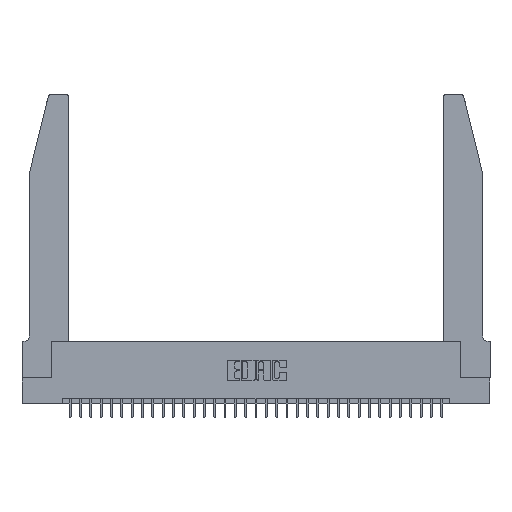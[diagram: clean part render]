
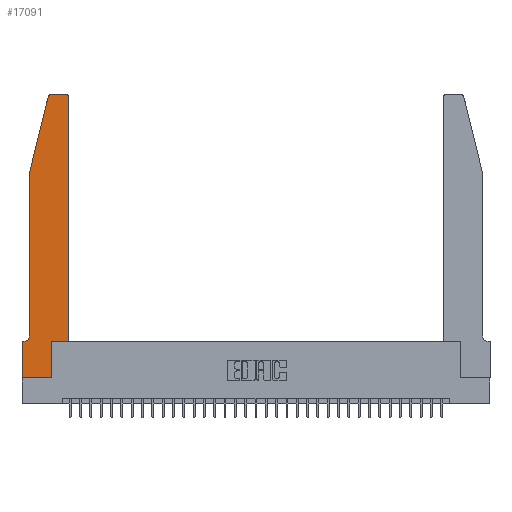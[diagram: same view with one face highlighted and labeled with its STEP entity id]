
A CAD part, top view. The second image highlights one B-rep face of the part: STEP entity #17091.
In plain terms, the highlighted planar face has unit normal (0, 0, 1).
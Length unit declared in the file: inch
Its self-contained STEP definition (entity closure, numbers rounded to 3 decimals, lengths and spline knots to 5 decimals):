
#749 = LINE ( 'NONE', #29789, #25771 ) ;
#884 = PLANE ( 'NONE',  #28031 ) ;
#921 = CARTESIAN_POINT ( 'NONE',  ( 0.4205, 2.72, 0.37 ) ) ;
#1233 = DIRECTION ( 'NONE',  ( 0., 0., 1. ) ) ;
#1353 = VECTOR ( 'NONE', #1467, 39.37008 ) ;
#1467 = DIRECTION ( 'NONE',  ( 0., -1., 0. ) ) ;
#1712 = ORIENTED_EDGE ( 'NONE', *, *, #6478, .T. ) ;
#1741 = CARTESIAN_POINT ( 'NONE',  ( 0., 0., 0.37 ) ) ;
#2584 = VERTEX_POINT ( 'NONE', #10958 ) ;
#2595 = ORIENTED_EDGE ( 'NONE', *, *, #30237, .T. ) ;
#3160 = VECTOR ( 'NONE', #19468, 39.37008 ) ;
#4023 = VERTEX_POINT ( 'NONE', #29581 ) ;
#4165 = ORIENTED_EDGE ( 'NONE', *, *, #14475, .T. ) ;
#5285 = VECTOR ( 'NONE', #31434, 39.37008 ) ;
#5296 = CARTESIAN_POINT ( 'NONE',  ( 0.4505, 0.35, 0.37 ) ) ;
#5356 = LINE ( 'NONE', #7424, #5285 ) ;
#5617 = ORIENTED_EDGE ( 'NONE', *, *, #32740, .T. ) ;
#5955 = VERTEX_POINT ( 'NONE', #13078 ) ;
#6478 = EDGE_CURVE ( 'NONE', #10735, #11610, #31607, .T. ) ;
#6593 = CIRCLE ( 'NONE', #11052, 0.07 ) ;
#6768 = CARTESIAN_POINT ( 'NONE',  ( 0.0755, 2., 0.37 ) ) ;
#6845 = ORIENTED_EDGE ( 'NONE', *, *, #18375, .T. ) ;
#7424 = CARTESIAN_POINT ( 'NONE',  ( 0., 0., 0.37 ) ) ;
#8068 = EDGE_CURVE ( 'NONE', #25461, #2584, #25272, .T. ) ;
#8406 = CARTESIAN_POINT ( 'NONE',  ( 0., 0., 0.37 ) ) ;
#8772 = LINE ( 'NONE', #8406, #3160 ) ;
#8917 = DIRECTION ( 'NONE',  ( 0., 0., 1. ) ) ;
#9054 = CARTESIAN_POINT ( 'NONE',  ( 0.2865, 0.35, 0.37 ) ) ;
#9136 = ORIENTED_EDGE ( 'NONE', *, *, #8068, .T. ) ;
#9634 = DIRECTION ( 'NONE',  ( 0., 0., -1. ) ) ;
#10425 = LINE ( 'NONE', #21261, #24882 ) ;
#10735 = VERTEX_POINT ( 'NONE', #19805 ) ;
#10795 = EDGE_CURVE ( 'NONE', #16302, #22369, #6593, .T. ) ;
#10958 = CARTESIAN_POINT ( 'NONE',  ( 0.25487, 2.72718, 0.37 ) ) ;
#11052 = AXIS2_PLACEMENT_3D ( 'NONE', #12244, #9634, #22392 ) ;
#11101 = VERTEX_POINT ( 'NONE', #6768 ) ;
#11190 = CARTESIAN_POINT ( 'NONE',  ( 0.4205, 2.75, 0.37 ) ) ;
#11448 = VECTOR ( 'NONE', #24638, 39.37008 ) ;
#11577 = DIRECTION ( 'NONE',  ( 0., 0., 1. ) ) ;
#11610 = VERTEX_POINT ( 'NONE', #11190 ) ;
#12244 = CARTESIAN_POINT ( 'NONE',  ( 0.0055, 0.42, 0.37 ) ) ;
#12999 = LINE ( 'NONE', #5296, #15747 ) ;
#13078 = CARTESIAN_POINT ( 'NONE',  ( 0.2865, 0., 0.37 ) ) ;
#14475 = EDGE_CURVE ( 'NONE', #26114, #4023, #12999, .T. ) ;
#14532 = DIRECTION ( 'NONE',  ( 1., 0., 0. ) ) ;
#15346 = EDGE_CURVE ( 'NONE', #22369, #16473, #23579, .T. ) ;
#15747 = VECTOR ( 'NONE', #31720, 39.37008 ) ;
#16057 = CARTESIAN_POINT ( 'NONE',  ( 0.0755, 0.42, 0.37 ) ) ;
#16302 = VERTEX_POINT ( 'NONE', #16057 ) ;
#16473 = VERTEX_POINT ( 'NONE', #32996 ) ;
#16662 = EDGE_CURVE ( 'NONE', #5955, #26114, #749, .T. ) ;
#17091 = ADVANCED_FACE ( 'NONE', ( #32904 ), #884, .T. ) ;
#17492 = DIRECTION ( 'NONE',  ( 1., 0., 0. ) ) ;
#17626 = ORIENTED_EDGE ( 'NONE', *, *, #29405, .T. ) ;
#18089 = AXIS2_PLACEMENT_3D ( 'NONE', #921, #11577, #30134 ) ;
#18313 = ORIENTED_EDGE ( 'NONE', *, *, #16662, .T. ) ;
#18375 = EDGE_CURVE ( 'NONE', #2584, #11101, #32875, .T. ) ;
#18906 = CARTESIAN_POINT ( 'NONE',  ( 0.4505, 0.35, 0.37 ) ) ;
#19468 = DIRECTION ( 'NONE',  ( 1., 0., 0. ) ) ;
#19798 = EDGE_CURVE ( 'NONE', #11101, #16302, #28036, .T. ) ;
#19805 = CARTESIAN_POINT ( 'NONE',  ( 0.4505, 2.72, 0.37 ) ) ;
#20952 = DIRECTION ( 'NONE',  ( -1., 0., 0. ) ) ;
#21128 = CARTESIAN_POINT ( 'NONE',  ( 0.0755, 0.35, 0.37 ) ) ;
#21261 = CARTESIAN_POINT ( 'NONE',  ( 0.2605, 2.75, 0.37 ) ) ;
#22349 = DIRECTION ( 'NONE',  ( -0.239, -0.971, 0. ) ) ;
#22369 = VERTEX_POINT ( 'NONE', #28706 ) ;
#22392 = DIRECTION ( 'NONE',  ( -1., 0., 0. ) ) ;
#23579 = LINE ( 'NONE', #21128, #25237 ) ;
#24131 = LINE ( 'NONE', #18906, #11448 ) ;
#24638 = DIRECTION ( 'NONE',  ( 0., 1., 0. ) ) ;
#24882 = VECTOR ( 'NONE', #34420, 39.37008 ) ;
#25176 = CARTESIAN_POINT ( 'NONE',  ( 0.284, 2.72, 0.37 ) ) ;
#25237 = VECTOR ( 'NONE', #20952, 39.37008 ) ;
#25239 = CARTESIAN_POINT ( 'NONE',  ( 0.0755, 2., 0.37 ) ) ;
#25272 = CIRCLE ( 'NONE', #29747, 0.03 ) ;
#25461 = VERTEX_POINT ( 'NONE', #30428 ) ;
#25683 = ORIENTED_EDGE ( 'NONE', *, *, #15346, .T. ) ;
#25771 = VECTOR ( 'NONE', #26799, 39.37008 ) ;
#26114 = VERTEX_POINT ( 'NONE', #9054 ) ;
#26799 = DIRECTION ( 'NONE',  ( 0., 1., 0. ) ) ;
#27226 = ORIENTED_EDGE ( 'NONE', *, *, #10795, .T. ) ;
#27533 = VECTOR ( 'NONE', #22349, 39.37008 ) ;
#27764 = CARTESIAN_POINT ( 'NONE',  ( 0.0755, 2., 0.37 ) ) ;
#27771 = ORIENTED_EDGE ( 'NONE', *, *, #19798, .T. ) ;
#27969 = CARTESIAN_POINT ( 'NONE',  ( 0., 0.35, 0.37 ) ) ;
#28031 = AXIS2_PLACEMENT_3D ( 'NONE', #27969, #8917, #14532 ) ;
#28036 = LINE ( 'NONE', #25239, #1353 ) ;
#28273 = EDGE_LOOP ( 'NONE', ( #5617, #9136, #6845, #27771, #27226, #25683, #17626, #28955, #18313, #4165, #2595, #1712 ) ) ;
#28706 = CARTESIAN_POINT ( 'NONE',  ( 0.0055, 0.35, 0.37 ) ) ;
#28955 = ORIENTED_EDGE ( 'NONE', *, *, #33451, .T. ) ;
#29030 = VERTEX_POINT ( 'NONE', #1741 ) ;
#29405 = EDGE_CURVE ( 'NONE', #16473, #29030, #5356, .T. ) ;
#29581 = CARTESIAN_POINT ( 'NONE',  ( 0.4505, 0.35, 0.37 ) ) ;
#29747 = AXIS2_PLACEMENT_3D ( 'NONE', #25176, #1233, #17492 ) ;
#29789 = CARTESIAN_POINT ( 'NONE',  ( 0.2865, 0.35, 0.37 ) ) ;
#30134 = DIRECTION ( 'NONE',  ( 1., 0., 0. ) ) ;
#30237 = EDGE_CURVE ( 'NONE', #4023, #10735, #24131, .T. ) ;
#30428 = CARTESIAN_POINT ( 'NONE',  ( 0.284, 2.75, 0.37 ) ) ;
#31434 = DIRECTION ( 'NONE',  ( 0., -1., 0. ) ) ;
#31607 = CIRCLE ( 'NONE', #18089, 0.03 ) ;
#31720 = DIRECTION ( 'NONE',  ( 1., 0., 0. ) ) ;
#32740 = EDGE_CURVE ( 'NONE', #11610, #25461, #10425, .T. ) ;
#32875 = LINE ( 'NONE', #27764, #27533 ) ;
#32904 = FACE_OUTER_BOUND ( 'NONE', #28273, .T. ) ;
#32996 = CARTESIAN_POINT ( 'NONE',  ( 0., 0.35, 0.37 ) ) ;
#33451 = EDGE_CURVE ( 'NONE', #29030, #5955, #8772, .T. ) ;
#34420 = DIRECTION ( 'NONE',  ( -1., 0., 0. ) ) ;
